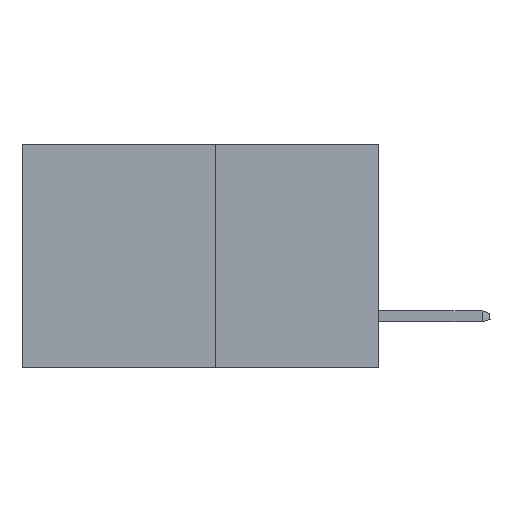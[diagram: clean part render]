
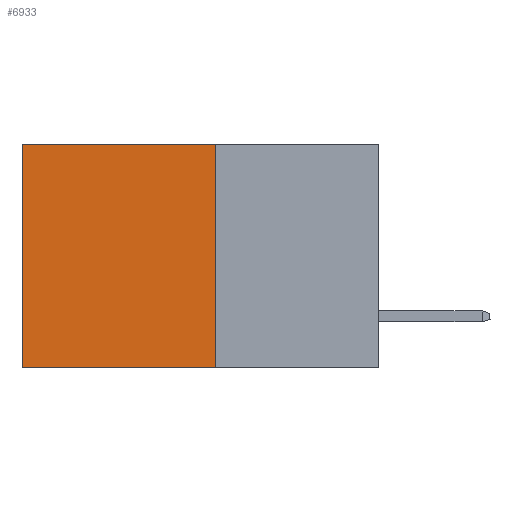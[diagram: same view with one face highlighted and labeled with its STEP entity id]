
A CAD part, left-side view. The second image highlights one B-rep face of the part: STEP entity #6933.
In plain terms, the highlighted planar face has unit normal (-1, 0, 0).
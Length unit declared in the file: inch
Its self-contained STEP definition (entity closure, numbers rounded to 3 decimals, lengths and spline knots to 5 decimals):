
#130 = CARTESIAN_POINT ( 'NONE',  ( 0.277, 0.27, 0. ) ) ;
#661 = ORIENTED_EDGE ( 'NONE', *, *, #13491, .T. ) ;
#960 = VERTEX_POINT ( 'NONE', #12707 ) ;
#1171 = FACE_OUTER_BOUND ( 'NONE', #13317, .T. ) ;
#1306 = PLANE ( 'NONE',  #3826 ) ;
#1645 = ORIENTED_EDGE ( 'NONE', *, *, #7364, .T. ) ;
#1921 = VERTEX_POINT ( 'NONE', #130 ) ;
#3327 = CARTESIAN_POINT ( 'NONE',  ( 0.277, 0.27, -0.37 ) ) ;
#3469 = CARTESIAN_POINT ( 'NONE',  ( 0.277, 0.27, 0. ) ) ;
#3744 = CARTESIAN_POINT ( 'NONE',  ( 0.277, 0.59, -0.37 ) ) ;
#3826 = AXIS2_PLACEMENT_3D ( 'NONE', #12172, #14477, #7447 ) ;
#3911 = CARTESIAN_POINT ( 'NONE',  ( 0.277, 0.27, -0.37 ) ) ;
#4649 = CARTESIAN_POINT ( 'NONE',  ( 0.277, 0.59, 0. ) ) ;
#5166 = VECTOR ( 'NONE', #13044, 39.37008 ) ;
#5284 = VERTEX_POINT ( 'NONE', #15094 ) ;
#5364 = ORIENTED_EDGE ( 'NONE', *, *, #12895, .F. ) ;
#6814 = LINE ( 'NONE', #3911, #9644 ) ;
#6933 = ADVANCED_FACE ( 'NONE', ( #1171 ), #1306, .F. ) ;
#7364 = EDGE_CURVE ( 'NONE', #10996, #5284, #11763, .T. ) ;
#7447 = DIRECTION ( 'NONE',  ( 0., 0., -1. ) ) ;
#9644 = VECTOR ( 'NONE', #12262, 39.37008 ) ;
#9808 = ORIENTED_EDGE ( 'NONE', *, *, #14845, .F. ) ;
#10559 = DIRECTION ( 'NONE',  ( 0., 0., -1. ) ) ;
#10956 = DIRECTION ( 'NONE',  ( 0., 0., -1. ) ) ;
#10996 = VERTEX_POINT ( 'NONE', #4649 ) ;
#11763 = LINE ( 'NONE', #3744, #14793 ) ;
#12172 = CARTESIAN_POINT ( 'NONE',  ( 0.277, 0.27, -0.37 ) ) ;
#12262 = DIRECTION ( 'NONE',  ( 0., 1., 0. ) ) ;
#12468 = VECTOR ( 'NONE', #10559, 39.37008 ) ;
#12707 = CARTESIAN_POINT ( 'NONE',  ( 0.277, 0.27, -0.37 ) ) ;
#12895 = EDGE_CURVE ( 'NONE', #1921, #960, #15467, .T. ) ;
#13044 = DIRECTION ( 'NONE',  ( 0., 1., 0. ) ) ;
#13317 = EDGE_LOOP ( 'NONE', ( #1645, #9808, #5364, #661 ) ) ;
#13491 = EDGE_CURVE ( 'NONE', #1921, #10996, #14572, .T. ) ;
#14477 = DIRECTION ( 'NONE',  ( 1., 0., 0. ) ) ;
#14572 = LINE ( 'NONE', #3469, #5166 ) ;
#14793 = VECTOR ( 'NONE', #10956, 39.37008 ) ;
#14845 = EDGE_CURVE ( 'NONE', #960, #5284, #6814, .T. ) ;
#15094 = CARTESIAN_POINT ( 'NONE',  ( 0.277, 0.59, -0.37 ) ) ;
#15467 = LINE ( 'NONE', #3327, #12468 ) ;
